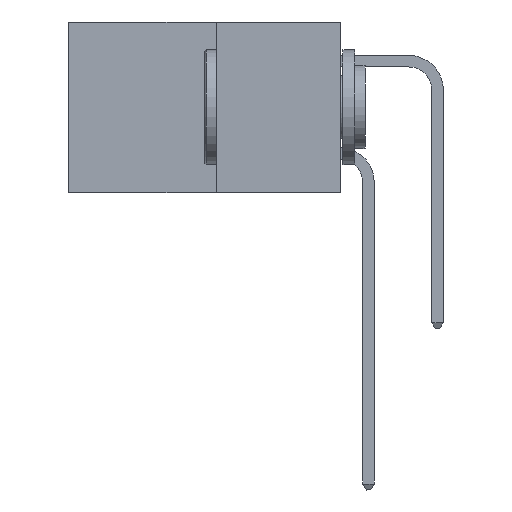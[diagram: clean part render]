
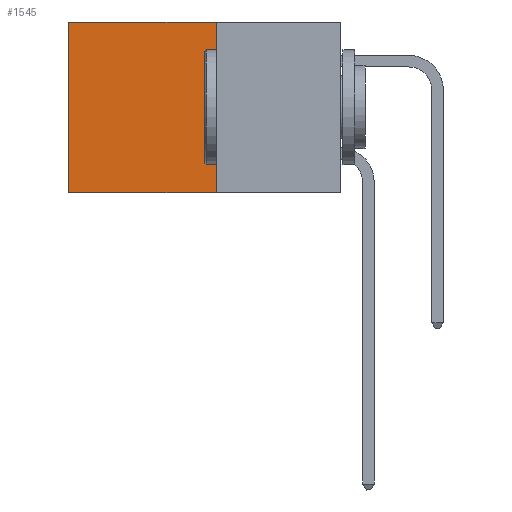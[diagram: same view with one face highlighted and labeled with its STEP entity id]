
A CAD part, left-side view. The second image highlights one B-rep face of the part: STEP entity #1545.
In plain terms, the highlighted planar face has unit normal (-1, 0, 0).
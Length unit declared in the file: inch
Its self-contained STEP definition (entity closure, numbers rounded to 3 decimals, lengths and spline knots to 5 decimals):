
#732 = VERTEX_POINT ( 'NONE', #10872 ) ;
#747 = DIRECTION ( 'NONE',  ( 0., 0., -1. ) ) ;
#1545 = ADVANCED_FACE ( 'NONE', ( #19830 ), #20267, .F. ) ;
#1800 = ORIENTED_EDGE ( 'NONE', *, *, #10218, .T. ) ;
#2002 = VERTEX_POINT ( 'NONE', #21442 ) ;
#2343 = VECTOR ( 'NONE', #21097, 39.37008 ) ;
#2576 = CARTESIAN_POINT ( 'NONE',  ( 0.277, 0.27, -0.37 ) ) ;
#2619 = EDGE_CURVE ( 'NONE', #20922, #11259, #21780, .T. ) ;
#5107 = CARTESIAN_POINT ( 'NONE',  ( 0.277, 0.59, -0.37 ) ) ;
#6920 = VECTOR ( 'NONE', #16324, 39.37008 ) ;
#7081 = VECTOR ( 'NONE', #15094, 39.37008 ) ;
#7735 = CARTESIAN_POINT ( 'NONE',  ( 0.277, 0.27, -0.37 ) ) ;
#8155 = VECTOR ( 'NONE', #747, 39.37008 ) ;
#8869 = EDGE_CURVE ( 'NONE', #2002, #732, #22805, .T. ) ;
#8978 = CARTESIAN_POINT ( 'NONE',  ( 0.277, 0.27, 0. ) ) ;
#9136 = ORIENTED_EDGE ( 'NONE', *, *, #22874, .F. ) ;
#9285 = DIRECTION ( 'NONE',  ( 1., 0., 0. ) ) ;
#10218 = EDGE_CURVE ( 'NONE', #2002, #20922, #22140, .T. ) ;
#10654 = CARTESIAN_POINT ( 'NONE',  ( 0.277, 0.59, 0. ) ) ;
#10872 = CARTESIAN_POINT ( 'NONE',  ( 0.277, 0.27, -0.37 ) ) ;
#11259 = VERTEX_POINT ( 'NONE', #5107 ) ;
#11953 = LINE ( 'NONE', #7735, #7081 ) ;
#12213 = EDGE_LOOP ( 'NONE', ( #21414, #9136, #23230, #1800 ) ) ;
#13815 = CARTESIAN_POINT ( 'NONE',  ( 0.277, 0.59, -0.37 ) ) ;
#14749 = CARTESIAN_POINT ( 'NONE',  ( 0.277, 0.27, -0.37 ) ) ;
#15094 = DIRECTION ( 'NONE',  ( 0., 1., 0. ) ) ;
#16324 = DIRECTION ( 'NONE',  ( 0., 1., 0. ) ) ;
#18761 = AXIS2_PLACEMENT_3D ( 'NONE', #14749, #9285, #22134 ) ;
#19830 = FACE_OUTER_BOUND ( 'NONE', #12213, .T. ) ;
#20267 = PLANE ( 'NONE',  #18761 ) ;
#20922 = VERTEX_POINT ( 'NONE', #10654 ) ;
#21097 = DIRECTION ( 'NONE',  ( 0., 0., -1. ) ) ;
#21414 = ORIENTED_EDGE ( 'NONE', *, *, #2619, .T. ) ;
#21442 = CARTESIAN_POINT ( 'NONE',  ( 0.277, 0.27, 0. ) ) ;
#21780 = LINE ( 'NONE', #13815, #2343 ) ;
#22134 = DIRECTION ( 'NONE',  ( 0., 0., -1. ) ) ;
#22140 = LINE ( 'NONE', #8978, #6920 ) ;
#22805 = LINE ( 'NONE', #2576, #8155 ) ;
#22874 = EDGE_CURVE ( 'NONE', #732, #11259, #11953, .T. ) ;
#23230 = ORIENTED_EDGE ( 'NONE', *, *, #8869, .F. ) ;
